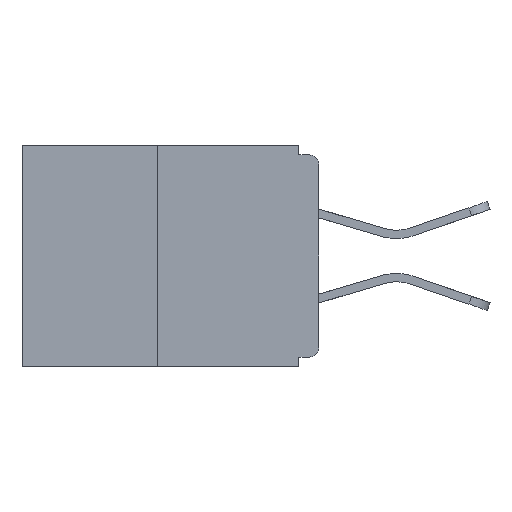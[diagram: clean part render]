
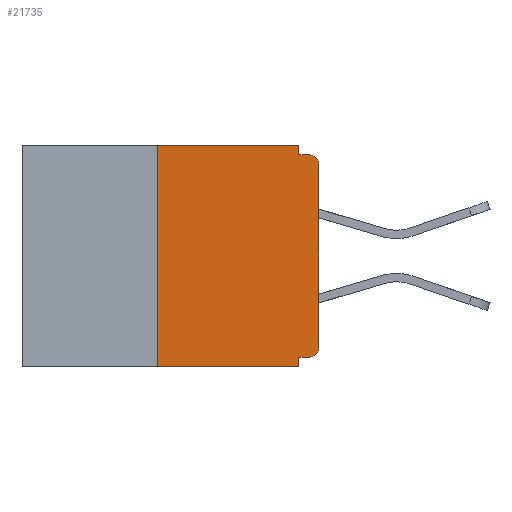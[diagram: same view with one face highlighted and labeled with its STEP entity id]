
A CAD part, left-side view. The second image highlights one B-rep face of the part: STEP entity #21735.
In plain terms, the highlighted planar face has unit normal (-1, 0, 0).
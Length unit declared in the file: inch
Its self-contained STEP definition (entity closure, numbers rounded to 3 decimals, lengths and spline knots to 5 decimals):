
#1232 = CARTESIAN_POINT ( 'NONE',  ( 0., 0.031, -0.343 ) ) ;
#1634 = CARTESIAN_POINT ( 'NONE',  ( 0., 0.015, -0.328 ) ) ;
#1661 = CARTESIAN_POINT ( 'NONE',  ( 0., 0.46, 0. ) ) ;
#2837 = CARTESIAN_POINT ( 'NONE',  ( 0., 0.015, -0.313 ) ) ;
#2931 = CARTESIAN_POINT ( 'NONE',  ( 0., 0.015, -0.015 ) ) ;
#3704 = LINE ( 'NONE', #20531, #23436 ) ;
#3771 = CIRCLE ( 'NONE', #4728, 0.015 ) ;
#3990 = VERTEX_POINT ( 'NONE', #15106 ) ;
#4502 = DIRECTION ( 'NONE',  ( -1., 0., 0. ) ) ;
#4560 = EDGE_CURVE ( 'NONE', #16002, #7407, #3771, .T. ) ;
#4728 = AXIS2_PLACEMENT_3D ( 'NONE', #23000, #4502, #29548 ) ;
#4845 = ORIENTED_EDGE ( 'NONE', *, *, #15349, .F. ) ;
#6347 = LINE ( 'NONE', #27124, #22941 ) ;
#6550 = PLANE ( 'NONE',  #14342 ) ;
#7020 = LINE ( 'NONE', #20488, #18861 ) ;
#7124 = DIRECTION ( 'NONE',  ( 0., 1., 0. ) ) ;
#7292 = VECTOR ( 'NONE', #7124, 39.37008 ) ;
#7338 = ORIENTED_EDGE ( 'NONE', *, *, #10806, .F. ) ;
#7407 = VERTEX_POINT ( 'NONE', #2931 ) ;
#8152 = VECTOR ( 'NONE', #15081, 39.37008 ) ;
#8856 = DIRECTION ( 'NONE',  ( 0., 0., -1. ) ) ;
#9411 = VERTEX_POINT ( 'NONE', #18182 ) ;
#9512 = ORIENTED_EDGE ( 'NONE', *, *, #20057, .F. ) ;
#9576 = ORIENTED_EDGE ( 'NONE', *, *, #29093, .T. ) ;
#9914 = VERTEX_POINT ( 'NONE', #24880 ) ;
#9955 = VERTEX_POINT ( 'NONE', #1634 ) ;
#10310 = DIRECTION ( 'NONE',  ( -1., 0., 0. ) ) ;
#10806 = EDGE_CURVE ( 'NONE', #9411, #11592, #7020, .T. ) ;
#11055 = EDGE_CURVE ( 'NONE', #21906, #9914, #26877, .T. ) ;
#11515 = VERTEX_POINT ( 'NONE', #15045 ) ;
#11517 = CARTESIAN_POINT ( 'NONE',  ( 0., 0.031, -0.015 ) ) ;
#11592 = VERTEX_POINT ( 'NONE', #11517 ) ;
#11671 = AXIS2_PLACEMENT_3D ( 'NONE', #2837, #10310, #21770 ) ;
#11812 = ORIENTED_EDGE ( 'NONE', *, *, #16359, .T. ) ;
#12345 = LINE ( 'NONE', #14899, #25738 ) ;
#12967 = ORIENTED_EDGE ( 'NONE', *, *, #19112, .F. ) ;
#13183 = DIRECTION ( 'NONE',  ( 0., 0., -1. ) ) ;
#13195 = CARTESIAN_POINT ( 'NONE',  ( 0., 0., -0.313 ) ) ;
#13644 = ORIENTED_EDGE ( 'NONE', *, *, #28651, .F. ) ;
#14342 = AXIS2_PLACEMENT_3D ( 'NONE', #1661, #15866, #20484 ) ;
#14899 = CARTESIAN_POINT ( 'NONE',  ( 0., 0.25, 0. ) ) ;
#15045 = CARTESIAN_POINT ( 'NONE',  ( 0., 0.25, 0. ) ) ;
#15081 = DIRECTION ( 'NONE',  ( 0., -1., 0. ) ) ;
#15106 = CARTESIAN_POINT ( 'NONE',  ( 0., 0.031, -0.328 ) ) ;
#15349 = EDGE_CURVE ( 'NONE', #11592, #7407, #21690, .T. ) ;
#15476 = EDGE_LOOP ( 'NONE', ( #12967, #27626, #24206, #9512, #13644, #11812, #9576, #21713, #4845, #7338 ) ) ;
#15866 = DIRECTION ( 'NONE',  ( 1., 0., 0. ) ) ;
#15993 = CARTESIAN_POINT ( 'NONE',  ( 0., 0., -0.03 ) ) ;
#16002 = VERTEX_POINT ( 'NONE', #15993 ) ;
#16359 = EDGE_CURVE ( 'NONE', #9955, #28079, #29700, .T. ) ;
#18182 = CARTESIAN_POINT ( 'NONE',  ( 0., 0.031, 0. ) ) ;
#18861 = VECTOR ( 'NONE', #8856, 39.37008 ) ;
#19112 = EDGE_CURVE ( 'NONE', #11515, #9411, #3704, .T. ) ;
#19372 = CARTESIAN_POINT ( 'NONE',  ( 0., 0.25, -0.343 ) ) ;
#19407 = DIRECTION ( 'NONE',  ( 0., -1., 0. ) ) ;
#20057 = EDGE_CURVE ( 'NONE', #3990, #9914, #26928, .T. ) ;
#20251 = DIRECTION ( 'NONE',  ( 0., 0., 1. ) ) ;
#20484 = DIRECTION ( 'NONE',  ( 0., 0., -1. ) ) ;
#20488 = CARTESIAN_POINT ( 'NONE',  ( 0., 0.031, 0. ) ) ;
#20531 = CARTESIAN_POINT ( 'NONE',  ( 0., 0.46, 0. ) ) ;
#20837 = EDGE_CURVE ( 'NONE', #21906, #11515, #12345, .T. ) ;
#20896 = CARTESIAN_POINT ( 'NONE',  ( 0., 0., -0.328 ) ) ;
#21061 = VECTOR ( 'NONE', #13183, 39.37008 ) ;
#21690 = LINE ( 'NONE', #22155, #29648 ) ;
#21713 = ORIENTED_EDGE ( 'NONE', *, *, #4560, .T. ) ;
#21735 = ADVANCED_FACE ( 'NONE', ( #25054 ), #6550, .F. ) ;
#21770 = DIRECTION ( 'NONE',  ( 0., 0., -1. ) ) ;
#21906 = VERTEX_POINT ( 'NONE', #19372 ) ;
#22155 = CARTESIAN_POINT ( 'NONE',  ( 0., 0., -0.015 ) ) ;
#22941 = VECTOR ( 'NONE', #20251, 39.37008 ) ;
#23000 = CARTESIAN_POINT ( 'NONE',  ( 0., 0.015, -0.03 ) ) ;
#23436 = VECTOR ( 'NONE', #26950, 39.37008 ) ;
#24104 = DIRECTION ( 'NONE',  ( 0., 0., 1. ) ) ;
#24206 = ORIENTED_EDGE ( 'NONE', *, *, #11055, .T. ) ;
#24880 = CARTESIAN_POINT ( 'NONE',  ( 0., 0.031, -0.343 ) ) ;
#25054 = FACE_OUTER_BOUND ( 'NONE', #15476, .T. ) ;
#25485 = LINE ( 'NONE', #20896, #7292 ) ;
#25738 = VECTOR ( 'NONE', #24104, 39.37008 ) ;
#26711 = CARTESIAN_POINT ( 'NONE',  ( 0., 0.46, -0.343 ) ) ;
#26877 = LINE ( 'NONE', #26711, #8152 ) ;
#26928 = LINE ( 'NONE', #1232, #21061 ) ;
#26950 = DIRECTION ( 'NONE',  ( 0., -1., 0. ) ) ;
#27124 = CARTESIAN_POINT ( 'NONE',  ( 0., 0., 0. ) ) ;
#27626 = ORIENTED_EDGE ( 'NONE', *, *, #20837, .F. ) ;
#28079 = VERTEX_POINT ( 'NONE', #13195 ) ;
#28651 = EDGE_CURVE ( 'NONE', #9955, #3990, #25485, .T. ) ;
#29093 = EDGE_CURVE ( 'NONE', #28079, #16002, #6347, .T. ) ;
#29548 = DIRECTION ( 'NONE',  ( 0., 0., -1. ) ) ;
#29648 = VECTOR ( 'NONE', #19407, 39.37008 ) ;
#29700 = CIRCLE ( 'NONE', #11671, 0.015 ) ;
